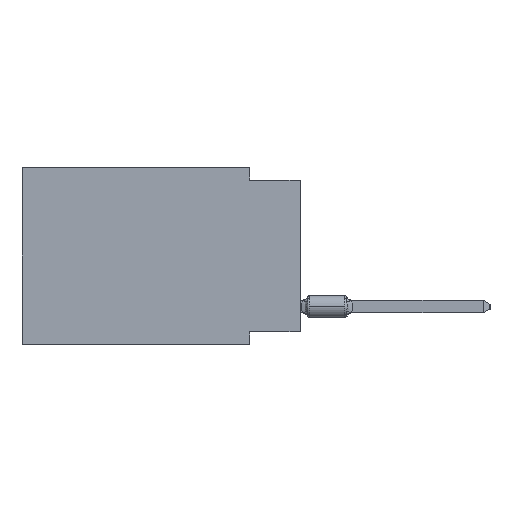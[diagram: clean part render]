
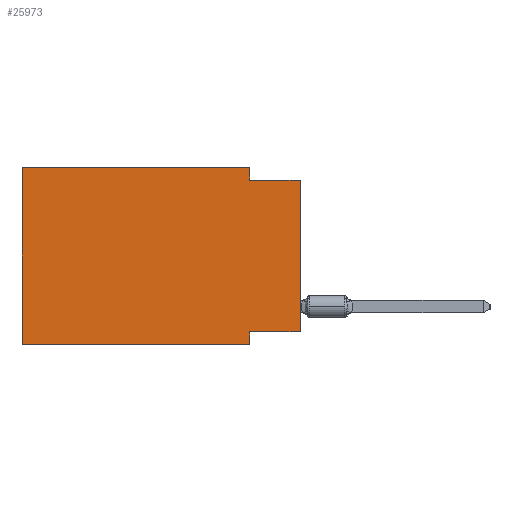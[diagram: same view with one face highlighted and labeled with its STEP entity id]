
A CAD part, left-side view. The second image highlights one B-rep face of the part: STEP entity #25973.
In plain terms, the highlighted planar face has unit normal (-1, 0, 0).
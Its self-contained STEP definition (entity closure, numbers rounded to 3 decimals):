
#1841 = DIRECTION ( 'NONE',  ( 0., 1., 0. ) ) ;
#2569 = ORIENTED_EDGE ( 'NONE', *, *, #82362, .F. ) ;
#9152 = ORIENTED_EDGE ( 'NONE', *, *, #98650, .F. ) ;
#10245 = FACE_OUTER_BOUND ( 'NONE', #28108, .T. ) ;
#10785 = CARTESIAN_POINT ( 'NONE',  ( 0., 13.97, 0. ) ) ;
#12166 = LINE ( 'NONE', #69313, #54770 ) ;
#13614 = ORIENTED_EDGE ( 'NONE', *, *, #69181, .F. ) ;
#14052 = VECTOR ( 'NONE', #46549, 1000. ) ;
#14724 = CARTESIAN_POINT ( 'NONE',  ( 0., 0., -8.255 ) ) ;
#17654 = CARTESIAN_POINT ( 'NONE',  ( 0., 13.97, -8.89 ) ) ;
#19839 = CARTESIAN_POINT ( 'NONE',  ( 0., 13.97, 0. ) ) ;
#20489 = VECTOR ( 'NONE', #76806, 1000. ) ;
#21033 = VERTEX_POINT ( 'NONE', #85143 ) ;
#21560 = LINE ( 'NONE', #23169, #33986 ) ;
#22526 = LINE ( 'NONE', #64286, #96788 ) ;
#22710 = VERTEX_POINT ( 'NONE', #73676 ) ;
#22817 = ORIENTED_EDGE ( 'NONE', *, *, #67563, .F. ) ;
#22952 = CARTESIAN_POINT ( 'NONE',  ( 0., 2.54, 0. ) ) ;
#23169 = CARTESIAN_POINT ( 'NONE',  ( 0., 0., 0. ) ) ;
#23688 = LINE ( 'NONE', #24239, #79860 ) ;
#24239 = CARTESIAN_POINT ( 'NONE',  ( 0., 0., -0.635 ) ) ;
#24506 = VERTEX_POINT ( 'NONE', #22952 ) ;
#25308 = ORIENTED_EDGE ( 'NONE', *, *, #56326, .T. ) ;
#25973 = ADVANCED_FACE ( 'NONE', ( #10245 ), #43744, .F. ) ;
#28108 = EDGE_LOOP ( 'NONE', ( #57207, #9152, #2569, #22817, #32700, #25308, #13614, #77459 ) ) ;
#29635 = CARTESIAN_POINT ( 'NONE',  ( 0., 13.97, 0. ) ) ;
#30349 = EDGE_CURVE ( 'NONE', #32853, #80345, #41992, .T. ) ;
#30706 = LINE ( 'NONE', #29635, #48956 ) ;
#31418 = DIRECTION ( 'NONE',  ( 0., 0., 1. ) ) ;
#32700 = ORIENTED_EDGE ( 'NONE', *, *, #55871, .F. ) ;
#32767 = CARTESIAN_POINT ( 'NONE',  ( 0., 2.54, -8.255 ) ) ;
#32853 = VERTEX_POINT ( 'NONE', #14724 ) ;
#33986 = VECTOR ( 'NONE', #31418, 1000. ) ;
#36880 = DIRECTION ( 'NONE',  ( 0., -1., 0. ) ) ;
#38654 = VERTEX_POINT ( 'NONE', #19839 ) ;
#40813 = VERTEX_POINT ( 'NONE', #105132 ) ;
#41992 = LINE ( 'NONE', #51826, #102561 ) ;
#42299 = VERTEX_POINT ( 'NONE', #17654 ) ;
#43744 = PLANE ( 'NONE',  #79120 ) ;
#46549 = DIRECTION ( 'NONE',  ( 0., 0., -1. ) ) ;
#48956 = VECTOR ( 'NONE', #88461, 1000. ) ;
#51514 = LINE ( 'NONE', #85067, #20489 ) ;
#51826 = CARTESIAN_POINT ( 'NONE',  ( 0., 0., -8.255 ) ) ;
#54770 = VECTOR ( 'NONE', #36880, 1000. ) ;
#55871 = EDGE_CURVE ( 'NONE', #42299, #38654, #22526, .T. ) ;
#56326 = EDGE_CURVE ( 'NONE', #42299, #21033, #12166, .T. ) ;
#57207 = ORIENTED_EDGE ( 'NONE', *, *, #104505, .T. ) ;
#57753 = DIRECTION ( 'NONE',  ( 0., -1., 0. ) ) ;
#64286 = CARTESIAN_POINT ( 'NONE',  ( 0., 13.97, 0. ) ) ;
#67563 = EDGE_CURVE ( 'NONE', #38654, #24506, #30706, .T. ) ;
#69181 = EDGE_CURVE ( 'NONE', #80345, #21033, #105904, .T. ) ;
#69313 = CARTESIAN_POINT ( 'NONE',  ( 0., 13.97, -8.89 ) ) ;
#73676 = CARTESIAN_POINT ( 'NONE',  ( 0., 0., -0.635 ) ) ;
#76806 = DIRECTION ( 'NONE',  ( 0., 0., -1. ) ) ;
#77459 = ORIENTED_EDGE ( 'NONE', *, *, #30349, .F. ) ;
#78399 = DIRECTION ( 'NONE',  ( 1., 0., 0. ) ) ;
#79120 = AXIS2_PLACEMENT_3D ( 'NONE', #10785, #78399, #103133 ) ;
#79860 = VECTOR ( 'NONE', #57753, 1000. ) ;
#80345 = VERTEX_POINT ( 'NONE', #32767 ) ;
#80803 = DIRECTION ( 'NONE',  ( 0., 0., 1. ) ) ;
#81187 = CARTESIAN_POINT ( 'NONE',  ( 0., 2.54, -8.89 ) ) ;
#82362 = EDGE_CURVE ( 'NONE', #24506, #40813, #51514, .T. ) ;
#85067 = CARTESIAN_POINT ( 'NONE',  ( 0., 2.54, 0. ) ) ;
#85143 = CARTESIAN_POINT ( 'NONE',  ( 0., 2.54, -8.89 ) ) ;
#88461 = DIRECTION ( 'NONE',  ( 0., -1., 0. ) ) ;
#96788 = VECTOR ( 'NONE', #80803, 1000. ) ;
#98650 = EDGE_CURVE ( 'NONE', #40813, #22710, #23688, .T. ) ;
#102561 = VECTOR ( 'NONE', #1841, 1000. ) ;
#103133 = DIRECTION ( 'NONE',  ( 0., 0., -1. ) ) ;
#104505 = EDGE_CURVE ( 'NONE', #32853, #22710, #21560, .T. ) ;
#105132 = CARTESIAN_POINT ( 'NONE',  ( 0., 2.54, -0.635 ) ) ;
#105904 = LINE ( 'NONE', #81187, #14052 ) ;
